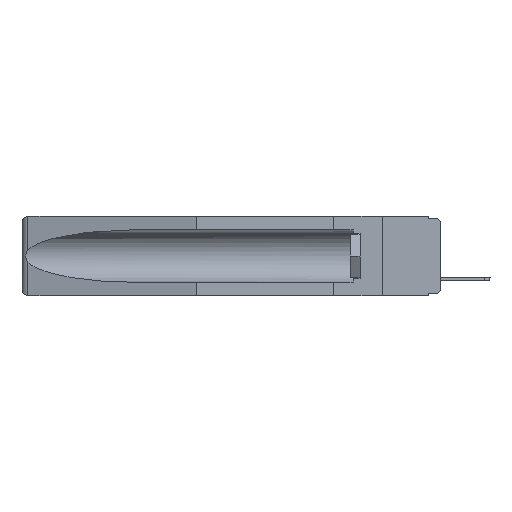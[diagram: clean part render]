
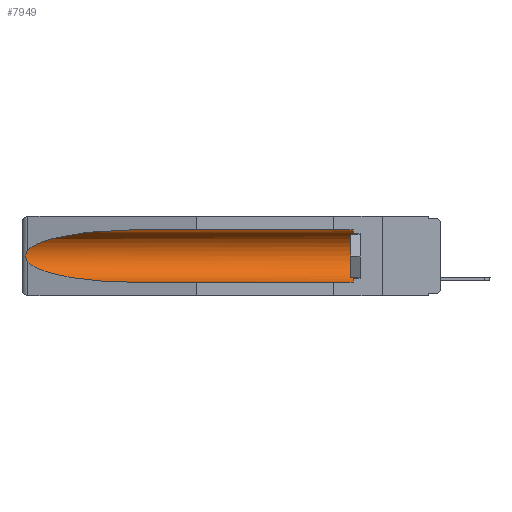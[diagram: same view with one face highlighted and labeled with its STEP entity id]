
A CAD part, left-side view. The second image highlights one B-rep face of the part: STEP entity #7949.
In plain terms, the highlighted cylindrical face has radius 2.857 mm (diameter 5.715 mm), a partial arc.
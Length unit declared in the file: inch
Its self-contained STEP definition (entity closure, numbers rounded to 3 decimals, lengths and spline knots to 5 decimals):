
#130 = VERTEX_POINT ( 'NONE', #18534 ) ;
#266 = ORIENTED_EDGE ( 'NONE', *, *, #17821, .T. ) ;
#654 = CARTESIAN_POINT ( 'NONE',  ( 0.26537, 1.52718, -0.14972 ) ) ;
#908 = CARTESIAN_POINT ( 'NONE',  ( 0.26537, 1.52718, -0.19328 ) ) ;
#1011 = LINE ( 'NONE', #11704, #12044 ) ;
#1604 = AXIS2_PLACEMENT_3D ( 'NONE', #11247, #7615, #20249 ) ;
#1942 = EDGE_CURVE ( 'NONE', #3848, #25203, #15287, .T. ) ;
#2703 = CARTESIAN_POINT ( 'NONE',  ( 0.26655, 1.53094, -0.18657 ) ) ;
#3177 = FACE_OUTER_BOUND ( 'NONE', #25612, .T. ) ;
#3700 = CARTESIAN_POINT ( 'NONE',  ( 0.155, 0.126, -0.059 ) ) ;
#3848 = VERTEX_POINT ( 'NONE', #12257 ) ;
#3895 = CARTESIAN_POINT ( 'NONE',  ( 0.155, 1.07973, -0.284 ) ) ;
#4342 = VERTEX_POINT ( 'NONE', #16384 ) ;
#5206 = EDGE_CURVE ( 'NONE', #3848, #9566, #10708, .T. ) ;
#7020 = B_SPLINE_CURVE_WITH_KNOTS ( 'NONE', 3,
 ( #7136, #7413, #17715, #7273, #20190, #13404, #18121, #2703, #20060, #908 ),
 .UNSPECIFIED., .F., .F.,
 ( 4, 2, 2, 2, 4 ),
 ( 0., 0.00029, 0.00058, 0.00087, 0.00117 ),
 .UNSPECIFIED. ) ;
#7136 = CARTESIAN_POINT ( 'NONE',  ( 0.26537, 1.52718, -0.14972 ) ) ;
#7273 = CARTESIAN_POINT ( 'NONE',  ( 0.2673, 1.5327, -0.16383 ) ) ;
#7296 = CARTESIAN_POINT ( 'NONE',  ( 0.155, 1.07973, -0.059 ) ) ;
#7413 = CARTESIAN_POINT ( 'NONE',  ( 0.26597, 1.52961, -0.15275 ) ) ;
#7615 = DIRECTION ( 'NONE',  ( 0., 1., 0. ) ) ;
#7887 = VECTOR ( 'NONE', #19185, 39.37008 ) ;
#7949 = ADVANCED_FACE ( 'NONE', ( #3177 ), #18175, .F. ) ;
#8372 = EDGE_CURVE ( 'NONE', #130, #11006, #14161, .T. ) ;
#9566 = VERTEX_POINT ( 'NONE', #3895 ) ;
#9976 = EDGE_CURVE ( 'NONE', #11006, #4342, #7020, .T. ) ;
#10357 = ORIENTED_EDGE ( 'NONE', *, *, #8372, .T. ) ;
#10435 = CARTESIAN_POINT ( 'NONE',  ( 0.155, 0.126, -0.1715 ) ) ;
#10708 = LINE ( 'NONE', #16824, #7887 ) ;
#11006 = VERTEX_POINT ( 'NONE', #26683 ) ;
#11247 = CARTESIAN_POINT ( 'NONE',  ( 0.155, -0.30754, -0.1715 ) ) ;
#11704 = CARTESIAN_POINT ( 'NONE',  ( 0.155, -0.30754, -0.059 ) ) ;
#12044 = VECTOR ( 'NONE', #26253, 39.37008 ) ;
#12257 = CARTESIAN_POINT ( 'NONE',  ( 0.155, 0.126, -0.284 ) ) ;
#12802 = EDGE_CURVE ( 'NONE', #25203, #130, #1011, .T. ) ;
#13278 =( BOUNDED_CURVE ( )  B_SPLINE_CURVE ( 3, ( #17403, #17820, #19471, #13365 ),
 .UNSPECIFIED., .F., .F. ) 
 B_SPLINE_CURVE_WITH_KNOTS ( ( 4, 4 ),
 ( 0.1948, 1.5708 ),
 .UNSPECIFIED. ) 
 CURVE ( )  GEOMETRIC_REPRESENTATION_ITEM ( )  RATIONAL_B_SPLINE_CURVE ( ( 1., 0.848, 0.848, 1. ) ) 
 REPRESENTATION_ITEM ( '' )  );
#13365 = CARTESIAN_POINT ( 'NONE',  ( 0.155, 1.07973, -0.284 ) ) ;
#13404 = CARTESIAN_POINT ( 'NONE',  ( 0.2675, 1.53308, -0.17534 ) ) ;
#14161 =( BOUNDED_CURVE ( )  B_SPLINE_CURVE ( 3, ( #7296, #19678, #15910, #654 ),
 .UNSPECIFIED., .F., .F. ) 
 B_SPLINE_CURVE_WITH_KNOTS ( ( 4, 4 ),
 ( 4.71239, 6.08839 ),
 .UNSPECIFIED. ) 
 CURVE ( )  GEOMETRIC_REPRESENTATION_ITEM ( )  RATIONAL_B_SPLINE_CURVE ( ( 1., 0.848, 0.848, 1. ) ) 
 REPRESENTATION_ITEM ( '' )  );
#14377 = ORIENTED_EDGE ( 'NONE', *, *, #9976, .T. ) ;
#15287 = CIRCLE ( 'NONE', #26381, 0.1125 ) ;
#15910 = CARTESIAN_POINT ( 'NONE',  ( 0.25451, 1.48313, -0.09465 ) ) ;
#16384 = CARTESIAN_POINT ( 'NONE',  ( 0.26537, 1.52718, -0.19328 ) ) ;
#16824 = CARTESIAN_POINT ( 'NONE',  ( 0.155, -0.30754, -0.284 ) ) ;
#16964 = DIRECTION ( 'NONE',  ( 0., 0., 1. ) ) ;
#17403 = CARTESIAN_POINT ( 'NONE',  ( 0.26537, 1.52718, -0.19328 ) ) ;
#17715 = CARTESIAN_POINT ( 'NONE',  ( 0.26654, 1.53092, -0.15636 ) ) ;
#17820 = CARTESIAN_POINT ( 'NONE',  ( 0.25451, 1.48313, -0.24835 ) ) ;
#17821 = EDGE_CURVE ( 'NONE', #4342, #9566, #13278, .T. ) ;
#18121 = CARTESIAN_POINT ( 'NONE',  ( 0.2673, 1.53269, -0.17917 ) ) ;
#18175 = CYLINDRICAL_SURFACE ( 'NONE', #1604, 0.1125 ) ;
#18534 = CARTESIAN_POINT ( 'NONE',  ( 0.155, 1.07973, -0.059 ) ) ;
#19036 = DIRECTION ( 'NONE',  ( 0., -1., 0. ) ) ;
#19185 = DIRECTION ( 'NONE',  ( 0., 1., 0. ) ) ;
#19471 = CARTESIAN_POINT ( 'NONE',  ( 0.21114, 1.30732, -0.284 ) ) ;
#19678 = CARTESIAN_POINT ( 'NONE',  ( 0.21114, 1.30732, -0.059 ) ) ;
#20060 = CARTESIAN_POINT ( 'NONE',  ( 0.26597, 1.5296, -0.19026 ) ) ;
#20190 = CARTESIAN_POINT ( 'NONE',  ( 0.2675, 1.53308, -0.16763 ) ) ;
#20249 = DIRECTION ( 'NONE',  ( 0., 0., 1. ) ) ;
#20467 = ORIENTED_EDGE ( 'NONE', *, *, #1942, .T. ) ;
#22373 = ORIENTED_EDGE ( 'NONE', *, *, #5206, .F. ) ;
#25203 = VERTEX_POINT ( 'NONE', #3700 ) ;
#25411 = ORIENTED_EDGE ( 'NONE', *, *, #12802, .T. ) ;
#25612 = EDGE_LOOP ( 'NONE', ( #10357, #14377, #266, #22373, #20467, #25411 ) ) ;
#26253 = DIRECTION ( 'NONE',  ( 0., 1., 0. ) ) ;
#26381 = AXIS2_PLACEMENT_3D ( 'NONE', #10435, #19036, #16964 ) ;
#26683 = CARTESIAN_POINT ( 'NONE',  ( 0.26537, 1.52718, -0.14972 ) ) ;
